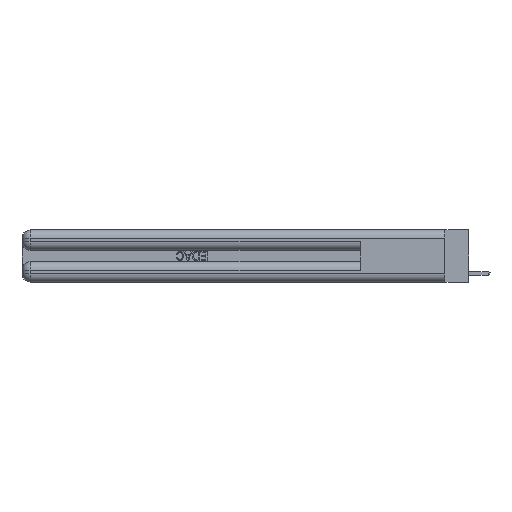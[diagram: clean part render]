
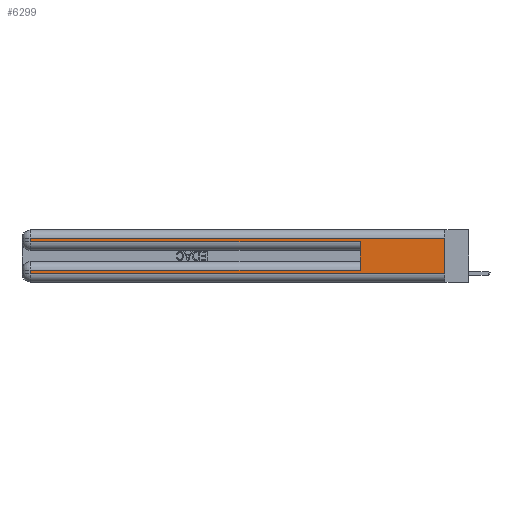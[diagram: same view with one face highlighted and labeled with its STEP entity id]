
A CAD part, left-side view. The second image highlights one B-rep face of the part: STEP entity #6299.
In plain terms, the highlighted planar face has unit normal (-1, 0, 0).
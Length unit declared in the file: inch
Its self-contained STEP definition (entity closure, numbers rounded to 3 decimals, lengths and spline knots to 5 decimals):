
#188 = VERTEX_POINT ( 'NONE', #15976 ) ;
#281 = ORIENTED_EDGE ( 'NONE', *, *, #24318, .T. ) ;
#355 = EDGE_CURVE ( 'NONE', #188, #3160, #26528, .T. ) ;
#374 = VECTOR ( 'NONE', #504, 39.37008 ) ;
#504 = DIRECTION ( 'NONE',  ( 0., 1., 0. ) ) ;
#1874 = DIRECTION ( 'NONE',  ( 0., -1., 0. ) ) ;
#2042 = VERTEX_POINT ( 'NONE', #21343 ) ;
#2598 = LINE ( 'NONE', #21341, #20263 ) ;
#2908 = VERTEX_POINT ( 'NONE', #24050 ) ;
#3160 = VERTEX_POINT ( 'NONE', #10139 ) ;
#3223 = LINE ( 'NONE', #17710, #20215 ) ;
#3510 = VERTEX_POINT ( 'NONE', #24387 ) ;
#4613 = DIRECTION ( 'NONE',  ( 0., -1., 0. ) ) ;
#4834 = LINE ( 'NONE', #6775, #374 ) ;
#5382 = LINE ( 'NONE', #17671, #21118 ) ;
#5391 = CARTESIAN_POINT ( 'NONE',  ( 0., 2.94, 0.37 ) ) ;
#6299 = ADVANCED_FACE ( 'NONE', ( #16189 ), #10208, .F. ) ;
#6775 = CARTESIAN_POINT ( 'NONE',  ( 0., 0., 0.31 ) ) ;
#6841 = VECTOR ( 'NONE', #15124, 39.37008 ) ;
#7475 = CARTESIAN_POINT ( 'NONE',  ( 0., 2.94, 0.285 ) ) ;
#7504 = VECTOR ( 'NONE', #4613, 39.37008 ) ;
#8209 = ORIENTED_EDGE ( 'NONE', *, *, #15269, .F. ) ;
#9566 = ORIENTED_EDGE ( 'NONE', *, *, #25791, .T. ) ;
#10139 = CARTESIAN_POINT ( 'NONE',  ( 0., 0., 0.06 ) ) ;
#10208 = PLANE ( 'NONE',  #11431 ) ;
#10406 = LINE ( 'NONE', #5391, #12386 ) ;
#11054 = EDGE_CURVE ( 'NONE', #20000, #15857, #15521, .T. ) ;
#11431 = AXIS2_PLACEMENT_3D ( 'NONE', #12463, #14533, #12169 ) ;
#12169 = DIRECTION ( 'NONE',  ( 0., 0., -1. ) ) ;
#12386 = VECTOR ( 'NONE', #25548, 39.37008 ) ;
#12463 = CARTESIAN_POINT ( 'NONE',  ( 0., 0., 0.37 ) ) ;
#12481 = VECTOR ( 'NONE', #20854, 39.37008 ) ;
#13266 = ORIENTED_EDGE ( 'NONE', *, *, #20377, .T. ) ;
#14402 = ORIENTED_EDGE ( 'NONE', *, *, #23786, .T. ) ;
#14533 = DIRECTION ( 'NONE',  ( 1., 0., 0. ) ) ;
#14880 = DIRECTION ( 'NONE',  ( 0., 0., -1. ) ) ;
#15058 = EDGE_LOOP ( 'NONE', ( #26418, #14402, #13266, #17034, #8209, #9566, #281, #19847 ) ) ;
#15124 = DIRECTION ( 'NONE',  ( 0., 0., 1. ) ) ;
#15269 = EDGE_CURVE ( 'NONE', #2908, #15857, #19685, .T. ) ;
#15521 = LINE ( 'NONE', #25387, #7504 ) ;
#15857 = VERTEX_POINT ( 'NONE', #24121 ) ;
#15976 = CARTESIAN_POINT ( 'NONE',  ( 0., 0., 0.31 ) ) ;
#16189 = FACE_OUTER_BOUND ( 'NONE', #15058, .T. ) ;
#16301 = CARTESIAN_POINT ( 'NONE',  ( 0., 0., 0.37 ) ) ;
#17034 = ORIENTED_EDGE ( 'NONE', *, *, #11054, .T. ) ;
#17671 = CARTESIAN_POINT ( 'NONE',  ( 0., 0., 0.085 ) ) ;
#17710 = CARTESIAN_POINT ( 'NONE',  ( 0., 2.94, 0.37 ) ) ;
#18896 = DIRECTION ( 'NONE',  ( 0., 1., 0. ) ) ;
#19685 = LINE ( 'NONE', #21101, #6841 ) ;
#19847 = ORIENTED_EDGE ( 'NONE', *, *, #23946, .T. ) ;
#20000 = VERTEX_POINT ( 'NONE', #7475 ) ;
#20215 = VECTOR ( 'NONE', #14880, 39.37008 ) ;
#20263 = VECTOR ( 'NONE', #1874, 39.37008 ) ;
#20377 = EDGE_CURVE ( 'NONE', #3510, #20000, #10406, .T. ) ;
#20854 = DIRECTION ( 'NONE',  ( 0., 0., -1. ) ) ;
#21101 = CARTESIAN_POINT ( 'NONE',  ( 0., 0.6, 0.145 ) ) ;
#21118 = VECTOR ( 'NONE', #18896, 39.37008 ) ;
#21341 = CARTESIAN_POINT ( 'NONE',  ( 0., 0., 0.06 ) ) ;
#21343 = CARTESIAN_POINT ( 'NONE',  ( 0., 2.94, 0.085 ) ) ;
#21744 = CARTESIAN_POINT ( 'NONE',  ( 0., 2.94, 0.06 ) ) ;
#23786 = EDGE_CURVE ( 'NONE', #188, #3510, #4834, .T. ) ;
#23946 = EDGE_CURVE ( 'NONE', #26384, #3160, #2598, .T. ) ;
#24050 = CARTESIAN_POINT ( 'NONE',  ( 0., 0.6, 0.085 ) ) ;
#24121 = CARTESIAN_POINT ( 'NONE',  ( 0., 0.6, 0.285 ) ) ;
#24318 = EDGE_CURVE ( 'NONE', #2042, #26384, #3223, .T. ) ;
#24387 = CARTESIAN_POINT ( 'NONE',  ( 0., 2.94, 0.31 ) ) ;
#25387 = CARTESIAN_POINT ( 'NONE',  ( 0., 0., 0.285 ) ) ;
#25548 = DIRECTION ( 'NONE',  ( 0., 0., -1. ) ) ;
#25791 = EDGE_CURVE ( 'NONE', #2908, #2042, #5382, .T. ) ;
#26384 = VERTEX_POINT ( 'NONE', #21744 ) ;
#26418 = ORIENTED_EDGE ( 'NONE', *, *, #355, .F. ) ;
#26528 = LINE ( 'NONE', #16301, #12481 ) ;
